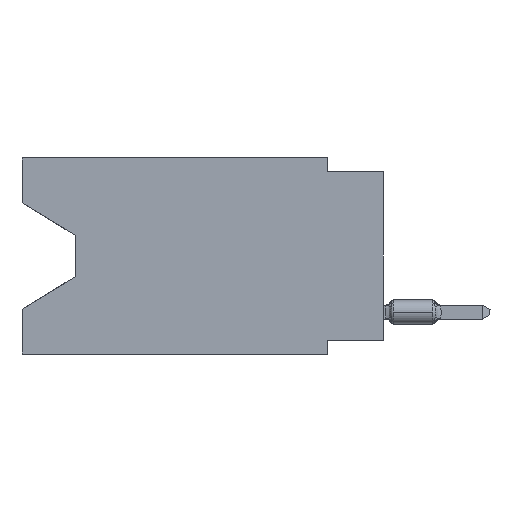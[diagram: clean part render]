
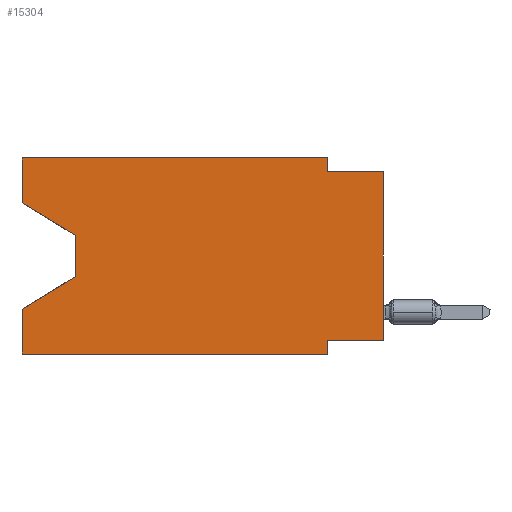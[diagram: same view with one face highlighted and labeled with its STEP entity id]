
A CAD part, left-side view. The second image highlights one B-rep face of the part: STEP entity #15304.
In plain terms, the highlighted planar face has unit normal (-1, 0, 0).
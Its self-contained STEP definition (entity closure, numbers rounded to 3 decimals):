
#45 = CARTESIAN_POINT ( 'NONE',  ( 0., 0., 0. ) ) ;
#357 = CARTESIAN_POINT ( 'NONE',  ( 0., 13.97, -3.505 ) ) ;
#622 = VERTEX_POINT ( 'NONE', #30070 ) ;
#749 = VECTOR ( 'NONE', #12172, 1000. ) ;
#2006 = ORIENTED_EDGE ( 'NONE', *, *, #6896, .F. ) ;
#2048 = CARTESIAN_POINT ( 'NONE',  ( 0., 13.97, -5.385 ) ) ;
#2276 = CARTESIAN_POINT ( 'NONE',  ( 0., 0., -0.635 ) ) ;
#4403 = CARTESIAN_POINT ( 'NONE',  ( 0., 2.54, 0. ) ) ;
#4833 = EDGE_CURVE ( 'NONE', #7358, #16352, #25658, .T. ) ;
#5450 = DIRECTION ( 'NONE',  ( 0., 0., -1. ) ) ;
#5657 = CARTESIAN_POINT ( 'NONE',  ( 0., 2.54, 0. ) ) ;
#5717 = ORIENTED_EDGE ( 'NONE', *, *, #31050, .T. ) ;
#5719 = DIRECTION ( 'NONE',  ( 0., 0., 1. ) ) ;
#6456 = VERTEX_POINT ( 'NONE', #13535 ) ;
#6764 = VERTEX_POINT ( 'NONE', #19837 ) ;
#6870 = VECTOR ( 'NONE', #27260, 1000. ) ;
#6896 = EDGE_CURVE ( 'NONE', #27613, #622, #10907, .T. ) ;
#6922 = CARTESIAN_POINT ( 'NONE',  ( 0., 16.383, -8.89 ) ) ;
#7358 = VERTEX_POINT ( 'NONE', #24587 ) ;
#7573 = VECTOR ( 'NONE', #11943, 1000. ) ;
#7610 = VECTOR ( 'NONE', #29287, 1000. ) ;
#7633 = CARTESIAN_POINT ( 'NONE',  ( 0., 16.383, 0. ) ) ;
#8299 = EDGE_CURVE ( 'NONE', #16352, #10719, #27576, .T. ) ;
#8421 = VERTEX_POINT ( 'NONE', #30485 ) ;
#8518 = VECTOR ( 'NONE', #27115, 1000. ) ;
#8634 = ORIENTED_EDGE ( 'NONE', *, *, #4833, .F. ) ;
#8989 = VECTOR ( 'NONE', #5719, 1000. ) ;
#9036 = VECTOR ( 'NONE', #24532, 1000. ) ;
#9570 = DIRECTION ( 'NONE',  ( 0., -0.855, -0.519 ) ) ;
#9728 = AXIS2_PLACEMENT_3D ( 'NONE', #20220, #27993, #5450 ) ;
#9938 = VECTOR ( 'NONE', #26138, 1000. ) ;
#10053 = LINE ( 'NONE', #14448, #17898 ) ;
#10163 = FACE_OUTER_BOUND ( 'NONE', #11248, .T. ) ;
#10259 = VECTOR ( 'NONE', #22423, 1000. ) ;
#10631 = ORIENTED_EDGE ( 'NONE', *, *, #8299, .F. ) ;
#10719 = VERTEX_POINT ( 'NONE', #4403 ) ;
#10907 = LINE ( 'NONE', #23391, #9938 ) ;
#10996 = CARTESIAN_POINT ( 'NONE',  ( 0., 13.97, -3.505 ) ) ;
#11248 = EDGE_LOOP ( 'NONE', ( #11994, #26719, #5717, #14151, #27788, #2006, #21970, #16982, #19930, #30793, #10631, #8634 ) ) ;
#11943 = DIRECTION ( 'NONE',  ( 0., 0.855, -0.519 ) ) ;
#11962 = LINE ( 'NONE', #6922, #7610 ) ;
#11994 = ORIENTED_EDGE ( 'NONE', *, *, #20070, .T. ) ;
#12010 = LINE ( 'NONE', #2276, #749 ) ;
#12172 = DIRECTION ( 'NONE',  ( 0., -1., 0. ) ) ;
#13535 = CARTESIAN_POINT ( 'NONE',  ( 0., 16.383, -8.89 ) ) ;
#13671 = VERTEX_POINT ( 'NONE', #10996 ) ;
#14151 = ORIENTED_EDGE ( 'NONE', *, *, #27452, .F. ) ;
#14267 = CARTESIAN_POINT ( 'NONE',  ( 0., 0., -8.255 ) ) ;
#14448 = CARTESIAN_POINT ( 'NONE',  ( 0., 16.383, -2.038 ) ) ;
#14631 = VERTEX_POINT ( 'NONE', #14267 ) ;
#14811 = LINE ( 'NONE', #45, #8518 ) ;
#15104 = EDGE_CURVE ( 'NONE', #6456, #622, #11962, .T. ) ;
#15304 = ADVANCED_FACE ( 'NONE', ( #10163 ), #27657, .F. ) ;
#15322 = VECTOR ( 'NONE', #27815, 1000. ) ;
#16352 = VERTEX_POINT ( 'NONE', #17470 ) ;
#16982 = ORIENTED_EDGE ( 'NONE', *, *, #28480, .T. ) ;
#17039 = LINE ( 'NONE', #5657, #31288 ) ;
#17195 = EDGE_CURVE ( 'NONE', #14631, #27613, #29212, .T. ) ;
#17470 = CARTESIAN_POINT ( 'NONE',  ( 0., 16.383, 0. ) ) ;
#17898 = VECTOR ( 'NONE', #9570, 1000. ) ;
#19668 = LINE ( 'NONE', #357, #9036 ) ;
#19837 = CARTESIAN_POINT ( 'NONE',  ( 0., 2.54, -0.635 ) ) ;
#19930 = ORIENTED_EDGE ( 'NONE', *, *, #28969, .F. ) ;
#20070 = EDGE_CURVE ( 'NONE', #7358, #13671, #10053, .T. ) ;
#20220 = CARTESIAN_POINT ( 'NONE',  ( 0., 16.383, 0. ) ) ;
#21828 = LINE ( 'NONE', #2048, #7573 ) ;
#21947 = CARTESIAN_POINT ( 'NONE',  ( 0., 0., -0.635 ) ) ;
#21970 = ORIENTED_EDGE ( 'NONE', *, *, #17195, .F. ) ;
#22423 = DIRECTION ( 'NONE',  ( 0., 1., 0. ) ) ;
#23247 = CARTESIAN_POINT ( 'NONE',  ( 0., 16.383, 0. ) ) ;
#23391 = CARTESIAN_POINT ( 'NONE',  ( 0., 2.54, -8.89 ) ) ;
#24532 = DIRECTION ( 'NONE',  ( 0., 0., -1. ) ) ;
#24587 = CARTESIAN_POINT ( 'NONE',  ( 0., 16.383, -2.038 ) ) ;
#24756 = LINE ( 'NONE', #25223, #15322 ) ;
#25223 = CARTESIAN_POINT ( 'NONE',  ( 0., 16.383, 0. ) ) ;
#25658 = LINE ( 'NONE', #23247, #8989 ) ;
#26021 = CARTESIAN_POINT ( 'NONE',  ( 0., 2.54, -8.255 ) ) ;
#26033 = VERTEX_POINT ( 'NONE', #30589 ) ;
#26138 = DIRECTION ( 'NONE',  ( 0., 0., -1. ) ) ;
#26719 = ORIENTED_EDGE ( 'NONE', *, *, #28508, .T. ) ;
#26784 = CARTESIAN_POINT ( 'NONE',  ( 0., 0., -8.255 ) ) ;
#27115 = DIRECTION ( 'NONE',  ( 0., 0., 1. ) ) ;
#27260 = DIRECTION ( 'NONE',  ( 0., -1., 0. ) ) ;
#27452 = EDGE_CURVE ( 'NONE', #6456, #26033, #24756, .T. ) ;
#27576 = LINE ( 'NONE', #7633, #6870 ) ;
#27613 = VERTEX_POINT ( 'NONE', #26021 ) ;
#27657 = PLANE ( 'NONE',  #9728 ) ;
#27788 = ORIENTED_EDGE ( 'NONE', *, *, #15104, .T. ) ;
#27815 = DIRECTION ( 'NONE',  ( 0., 0., 1. ) ) ;
#27993 = DIRECTION ( 'NONE',  ( 1., 0., 0. ) ) ;
#28194 = DIRECTION ( 'NONE',  ( 0., 0., -1. ) ) ;
#28480 = EDGE_CURVE ( 'NONE', #14631, #30166, #14811, .T. ) ;
#28508 = EDGE_CURVE ( 'NONE', #13671, #8421, #19668, .T. ) ;
#28969 = EDGE_CURVE ( 'NONE', #6764, #30166, #12010, .T. ) ;
#29048 = EDGE_CURVE ( 'NONE', #10719, #6764, #17039, .T. ) ;
#29212 = LINE ( 'NONE', #26784, #10259 ) ;
#29287 = DIRECTION ( 'NONE',  ( 0., -1., 0. ) ) ;
#30070 = CARTESIAN_POINT ( 'NONE',  ( 0., 2.54, -8.89 ) ) ;
#30166 = VERTEX_POINT ( 'NONE', #21947 ) ;
#30485 = CARTESIAN_POINT ( 'NONE',  ( 0., 13.97, -5.385 ) ) ;
#30589 = CARTESIAN_POINT ( 'NONE',  ( 0., 16.383, -6.852 ) ) ;
#30793 = ORIENTED_EDGE ( 'NONE', *, *, #29048, .F. ) ;
#31050 = EDGE_CURVE ( 'NONE', #8421, #26033, #21828, .T. ) ;
#31288 = VECTOR ( 'NONE', #28194, 1000. ) ;
